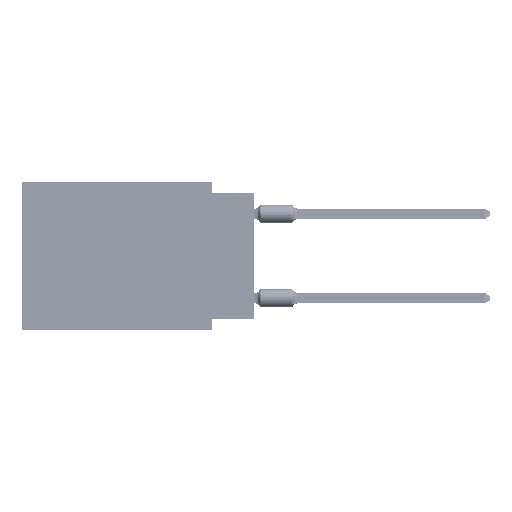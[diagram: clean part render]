
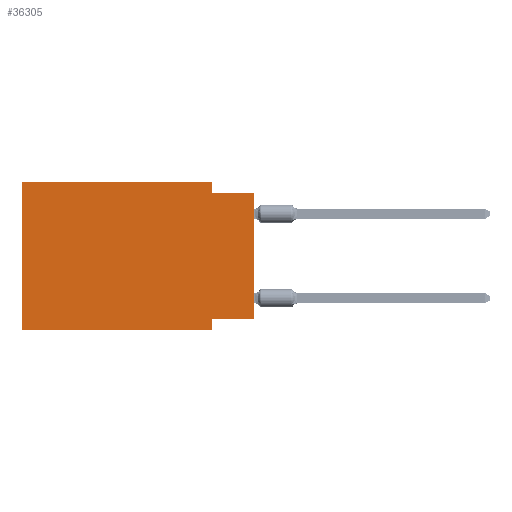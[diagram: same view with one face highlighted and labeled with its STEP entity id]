
A CAD part, left-side view. The second image highlights one B-rep face of the part: STEP entity #36305.
In plain terms, the highlighted planar face has unit normal (-1, 0, 0).
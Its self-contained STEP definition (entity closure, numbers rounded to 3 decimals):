
#961 = LINE ( 'NONE', #67607, #13401 ) ;
#2141 = VERTEX_POINT ( 'NONE', #47726 ) ;
#2724 = VERTEX_POINT ( 'NONE', #55937 ) ;
#4402 = EDGE_CURVE ( 'NONE', #77811, #74999, #50669, .T. ) ;
#5763 = CARTESIAN_POINT ( 'NONE',  ( 0., 13.97, 0. ) ) ;
#6534 = VECTOR ( 'NONE', #61104, 1000. ) ;
#7240 = CARTESIAN_POINT ( 'NONE',  ( 0., 13.97, -8.89 ) ) ;
#7298 = DIRECTION ( 'NONE',  ( 0., 0., 1. ) ) ;
#7963 = EDGE_CURVE ( 'NONE', #69676, #49223, #66976, .T. ) ;
#8760 = VERTEX_POINT ( 'NONE', #40202 ) ;
#9126 = ORIENTED_EDGE ( 'NONE', *, *, #25778, .T. ) ;
#9767 = CARTESIAN_POINT ( 'NONE',  ( 0., 0., -0.635 ) ) ;
#9971 = EDGE_CURVE ( 'NONE', #53435, #8760, #28794, .T. ) ;
#10335 = AXIS2_PLACEMENT_3D ( 'NONE', #5763, #78354, #23614 ) ;
#12230 = CARTESIAN_POINT ( 'NONE',  ( 0., 0., -8.255 ) ) ;
#13056 = ORIENTED_EDGE ( 'NONE', *, *, #73288, .T. ) ;
#13401 = VECTOR ( 'NONE', #7298, 1000. ) ;
#14452 = VECTOR ( 'NONE', #32824, 1000. ) ;
#14524 = EDGE_CURVE ( 'NONE', #2724, #77811, #961, .T. ) ;
#15074 = CARTESIAN_POINT ( 'NONE',  ( 0., 0., 0. ) ) ;
#15764 = CARTESIAN_POINT ( 'NONE',  ( 0., 2.54, -8.89 ) ) ;
#18188 = DIRECTION ( 'NONE',  ( 0., 1., 0. ) ) ;
#20361 = ORIENTED_EDGE ( 'NONE', *, *, #9971, .F. ) ;
#22777 = CARTESIAN_POINT ( 'NONE',  ( 0., 13.97, 0. ) ) ;
#23614 = DIRECTION ( 'NONE',  ( 0., 0., -1. ) ) ;
#25778 = EDGE_CURVE ( 'NONE', #69676, #8760, #57132, .T. ) ;
#26156 = VECTOR ( 'NONE', #18188, 1000. ) ;
#27645 = DIRECTION ( 'NONE',  ( 0., 0., -1. ) ) ;
#28794 = LINE ( 'NONE', #9767, #36546 ) ;
#31432 = LINE ( 'NONE', #7240, #77644 ) ;
#31736 = CARTESIAN_POINT ( 'NONE',  ( 0., 2.54, 0. ) ) ;
#32131 = LINE ( 'NONE', #31736, #6534 ) ;
#32824 = DIRECTION ( 'NONE',  ( 0., -1., 0. ) ) ;
#32881 = ORIENTED_EDGE ( 'NONE', *, *, #69669, .F. ) ;
#34050 = EDGE_LOOP ( 'NONE', ( #9126, #20361, #32881, #51215, #69928, #13056, #77643, #67790 ) ) ;
#35447 = CARTESIAN_POINT ( 'NONE',  ( 0., 2.54, 0. ) ) ;
#36305 = ADVANCED_FACE ( 'NONE', ( #65673 ), #60114, .F. ) ;
#36546 = VECTOR ( 'NONE', #70848, 1000. ) ;
#40202 = CARTESIAN_POINT ( 'NONE',  ( 0., 0., -0.635 ) ) ;
#40413 = EDGE_CURVE ( 'NONE', #49223, #2141, #45507, .T. ) ;
#44331 = CARTESIAN_POINT ( 'NONE',  ( 0., 13.97, 0. ) ) ;
#45507 = LINE ( 'NONE', #15764, #74204 ) ;
#47726 = CARTESIAN_POINT ( 'NONE',  ( 0., 2.54, -8.89 ) ) ;
#48308 = CARTESIAN_POINT ( 'NONE',  ( 0., 2.54, -0.635 ) ) ;
#49223 = VERTEX_POINT ( 'NONE', #54815 ) ;
#50669 = LINE ( 'NONE', #44331, #14452 ) ;
#51181 = DIRECTION ( 'NONE',  ( 0., 0., 1. ) ) ;
#51215 = ORIENTED_EDGE ( 'NONE', *, *, #4402, .F. ) ;
#51340 = VECTOR ( 'NONE', #51181, 1000. ) ;
#53435 = VERTEX_POINT ( 'NONE', #48308 ) ;
#54815 = CARTESIAN_POINT ( 'NONE',  ( 0., 2.54, -8.255 ) ) ;
#55937 = CARTESIAN_POINT ( 'NONE',  ( 0., 13.97, -8.89 ) ) ;
#56413 = DIRECTION ( 'NONE',  ( 0., -1., 0. ) ) ;
#57132 = LINE ( 'NONE', #15074, #51340 ) ;
#60114 = PLANE ( 'NONE',  #10335 ) ;
#61104 = DIRECTION ( 'NONE',  ( 0., 0., -1. ) ) ;
#61883 = CARTESIAN_POINT ( 'NONE',  ( 0., 0., -8.255 ) ) ;
#65673 = FACE_OUTER_BOUND ( 'NONE', #34050, .T. ) ;
#66976 = LINE ( 'NONE', #12230, #26156 ) ;
#67607 = CARTESIAN_POINT ( 'NONE',  ( 0., 13.97, 0. ) ) ;
#67790 = ORIENTED_EDGE ( 'NONE', *, *, #7963, .F. ) ;
#69669 = EDGE_CURVE ( 'NONE', #74999, #53435, #32131, .T. ) ;
#69676 = VERTEX_POINT ( 'NONE', #61883 ) ;
#69928 = ORIENTED_EDGE ( 'NONE', *, *, #14524, .F. ) ;
#70848 = DIRECTION ( 'NONE',  ( 0., -1., 0. ) ) ;
#73288 = EDGE_CURVE ( 'NONE', #2724, #2141, #31432, .T. ) ;
#74204 = VECTOR ( 'NONE', #27645, 1000. ) ;
#74999 = VERTEX_POINT ( 'NONE', #35447 ) ;
#77643 = ORIENTED_EDGE ( 'NONE', *, *, #40413, .F. ) ;
#77644 = VECTOR ( 'NONE', #56413, 1000. ) ;
#77811 = VERTEX_POINT ( 'NONE', #22777 ) ;
#78354 = DIRECTION ( 'NONE',  ( 1., 0., 0. ) ) ;
